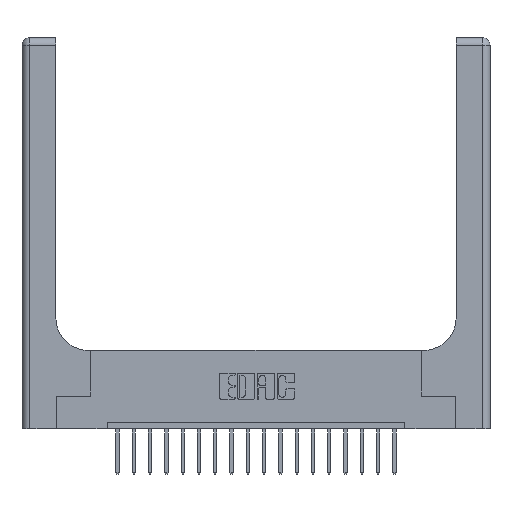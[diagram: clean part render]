
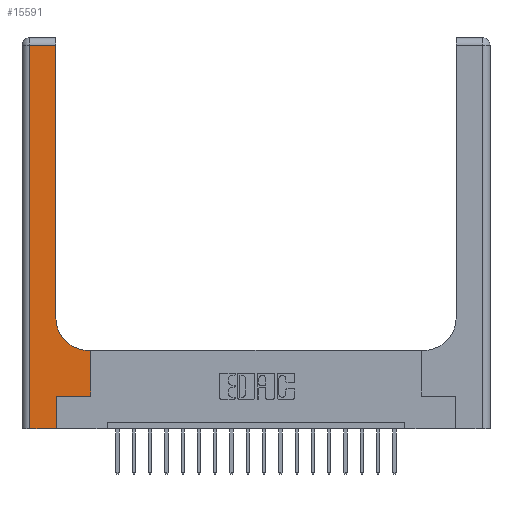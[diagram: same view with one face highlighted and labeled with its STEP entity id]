
A CAD part, top view. The second image highlights one B-rep face of the part: STEP entity #15591.
In plain terms, the highlighted planar face has unit normal (0, 0, 1).
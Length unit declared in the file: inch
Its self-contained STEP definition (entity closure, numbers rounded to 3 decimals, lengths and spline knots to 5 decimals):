
#108 = CARTESIAN_POINT ( 'NONE',  ( 0.26, 0.6, 0.37 ) ) ;
#1026 = ORIENTED_EDGE ( 'NONE', *, *, #10382, .T. ) ;
#1084 = ORIENTED_EDGE ( 'NONE', *, *, #9701, .T. ) ;
#1334 = VERTEX_POINT ( 'NONE', #9516 ) ;
#1375 = EDGE_CURVE ( 'NONE', #16136, #7978, #12714, .T. ) ;
#1498 = CARTESIAN_POINT ( 'NONE',  ( 0.51, 0.85, 0.37 ) ) ;
#1729 = CARTESIAN_POINT ( 'NONE',  ( 0., 3., 0.37 ) ) ;
#1956 = CARTESIAN_POINT ( 'NONE',  ( 0.06, 2.94, 0.37 ) ) ;
#2144 = DIRECTION ( 'NONE',  ( -1., 0., 0. ) ) ;
#2408 = VECTOR ( 'NONE', #5234, 39.37008 ) ;
#2851 = VECTOR ( 'NONE', #5195, 39.37008 ) ;
#2876 = LINE ( 'NONE', #3725, #2408 ) ;
#2952 = AXIS2_PLACEMENT_3D ( 'NONE', #1498, #4384, #8851 ) ;
#3616 = EDGE_CURVE ( 'NONE', #9216, #1334, #14365, .T. ) ;
#3725 = CARTESIAN_POINT ( 'NONE',  ( 0.26, 3., 0.37 ) ) ;
#4384 = DIRECTION ( 'NONE',  ( 0., 0., -1. ) ) ;
#4859 = DIRECTION ( 'NONE',  ( -1., 0., 0. ) ) ;
#5038 = VECTOR ( 'NONE', #9085, 39.37008 ) ;
#5195 = DIRECTION ( 'NONE',  ( 1., 0., 0. ) ) ;
#5234 = DIRECTION ( 'NONE',  ( 0., 1., 0. ) ) ;
#5617 = EDGE_CURVE ( 'NONE', #14324, #6604, #11592, .T. ) ;
#6063 = ORIENTED_EDGE ( 'NONE', *, *, #1375, .T. ) ;
#6604 = VERTEX_POINT ( 'NONE', #18979 ) ;
#6988 = CARTESIAN_POINT ( 'NONE',  ( 0.26, 2.94, 0.37 ) ) ;
#7350 = CARTESIAN_POINT ( 'NONE',  ( 0.265, 0., 0.37 ) ) ;
#7496 = CARTESIAN_POINT ( 'NONE',  ( 0.528, 0.25, 0.37 ) ) ;
#7978 = VERTEX_POINT ( 'NONE', #16112 ) ;
#8205 = DIRECTION ( 'NONE',  ( 0., 1., 0. ) ) ;
#8534 = ORIENTED_EDGE ( 'NONE', *, *, #14161, .T. ) ;
#8851 = DIRECTION ( 'NONE',  ( 1., 0., 0. ) ) ;
#8860 = LINE ( 'NONE', #108, #15388 ) ;
#9085 = DIRECTION ( 'NONE',  ( 1., 0., 0. ) ) ;
#9216 = VERTEX_POINT ( 'NONE', #12919 ) ;
#9294 = CARTESIAN_POINT ( 'NONE',  ( 0.528, 0.6, 0.37 ) ) ;
#9321 = ORIENTED_EDGE ( 'NONE', *, *, #13085, .T. ) ;
#9370 = DIRECTION ( 'NONE',  ( 0., 0., -1. ) ) ;
#9516 = CARTESIAN_POINT ( 'NONE',  ( 0.26, 0.85, 0.37 ) ) ;
#9593 = DIRECTION ( 'NONE',  ( 0., -1., 0. ) ) ;
#9596 = CARTESIAN_POINT ( 'NONE',  ( 0., 2.94, 0.37 ) ) ;
#9701 = EDGE_CURVE ( 'NONE', #7978, #14324, #13255, .T. ) ;
#9703 = CARTESIAN_POINT ( 'NONE',  ( 0.265, 0., 0.37 ) ) ;
#9721 = LINE ( 'NONE', #11607, #2851 ) ;
#10149 = AXIS2_PLACEMENT_3D ( 'NONE', #1729, #9370, #4859 ) ;
#10176 = DIRECTION ( 'NONE',  ( 0., 1., 0. ) ) ;
#10382 = EDGE_CURVE ( 'NONE', #10690, #16136, #10446, .T. ) ;
#10446 = LINE ( 'NONE', #9596, #18046 ) ;
#10683 = EDGE_CURVE ( 'NONE', #6604, #13066, #9721, .T. ) ;
#10690 = VERTEX_POINT ( 'NONE', #6988 ) ;
#10789 = DIRECTION ( 'NONE',  ( -1., 0., 0. ) ) ;
#10911 = ORIENTED_EDGE ( 'NONE', *, *, #5617, .T. ) ;
#10977 = EDGE_LOOP ( 'NONE', ( #8534, #1026, #6063, #1084, #10911, #12106, #11538, #9321, #11186 ) ) ;
#11186 = ORIENTED_EDGE ( 'NONE', *, *, #3616, .T. ) ;
#11538 = ORIENTED_EDGE ( 'NONE', *, *, #13186, .T. ) ;
#11592 = LINE ( 'NONE', #9703, #18672 ) ;
#11607 = CARTESIAN_POINT ( 'NONE',  ( 0.265, 0.25, 0.37 ) ) ;
#11747 = VECTOR ( 'NONE', #8205, 39.37008 ) ;
#12106 = ORIENTED_EDGE ( 'NONE', *, *, #10683, .T. ) ;
#12344 = CARTESIAN_POINT ( 'NONE',  ( 0., 0., 0.37 ) ) ;
#12714 = LINE ( 'NONE', #14470, #14800 ) ;
#12764 = VERTEX_POINT ( 'NONE', #9294 ) ;
#12912 = FACE_OUTER_BOUND ( 'NONE', #10977, .T. ) ;
#12919 = CARTESIAN_POINT ( 'NONE',  ( 0.51, 0.6, 0.37 ) ) ;
#13066 = VERTEX_POINT ( 'NONE', #7496 ) ;
#13085 = EDGE_CURVE ( 'NONE', #12764, #9216, #8860, .T. ) ;
#13186 = EDGE_CURVE ( 'NONE', #13066, #12764, #15541, .T. ) ;
#13255 = LINE ( 'NONE', #12344, #5038 ) ;
#14161 = EDGE_CURVE ( 'NONE', #1334, #10690, #2876, .T. ) ;
#14324 = VERTEX_POINT ( 'NONE', #7350 ) ;
#14365 = CIRCLE ( 'NONE', #2952, 0.25 ) ;
#14470 = CARTESIAN_POINT ( 'NONE',  ( 0.06, 3., 0.37 ) ) ;
#14800 = VECTOR ( 'NONE', #9593, 39.37008 ) ;
#15388 = VECTOR ( 'NONE', #10789, 39.37008 ) ;
#15541 = LINE ( 'NONE', #17357, #11747 ) ;
#15591 = ADVANCED_FACE ( 'NONE', ( #12912 ), #16880, .F. ) ;
#16112 = CARTESIAN_POINT ( 'NONE',  ( 0.06, 0., 0.37 ) ) ;
#16136 = VERTEX_POINT ( 'NONE', #1956 ) ;
#16880 = PLANE ( 'NONE',  #10149 ) ;
#17357 = CARTESIAN_POINT ( 'NONE',  ( 0.528, 0.25, 0.37 ) ) ;
#18046 = VECTOR ( 'NONE', #2144, 39.37008 ) ;
#18672 = VECTOR ( 'NONE', #10176, 39.37008 ) ;
#18979 = CARTESIAN_POINT ( 'NONE',  ( 0.265, 0.25, 0.37 ) ) ;
